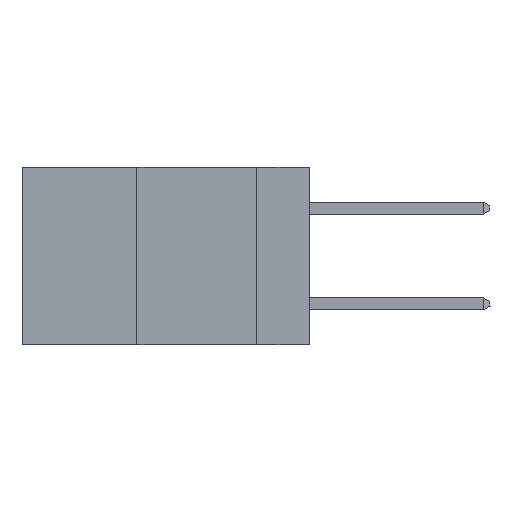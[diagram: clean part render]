
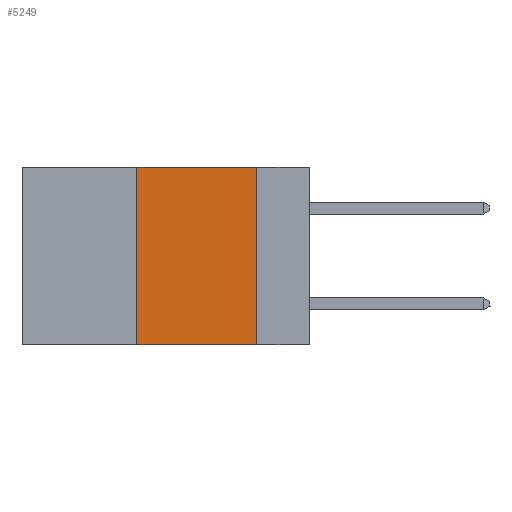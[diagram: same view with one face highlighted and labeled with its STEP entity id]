
A CAD part, left-side view. The second image highlights one B-rep face of the part: STEP entity #5249.
In plain terms, the highlighted planar face has unit normal (-1, 0, 0).
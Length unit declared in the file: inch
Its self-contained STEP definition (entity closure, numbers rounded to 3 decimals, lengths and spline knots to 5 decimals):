
#216 = AXIS2_PLACEMENT_3D ( 'NONE', #523, #10681, #2516 ) ;
#227 = CARTESIAN_POINT ( 'NONE',  ( 0., 0.36, 0. ) ) ;
#523 = CARTESIAN_POINT ( 'NONE',  ( 0., 0.6, 0. ) ) ;
#568 = VECTOR ( 'NONE', #9889, 39.37008 ) ;
#1484 = CARTESIAN_POINT ( 'NONE',  ( 0., 0.36, -0.37 ) ) ;
#1761 = DIRECTION ( 'NONE',  ( 0., 0., 1. ) ) ;
#1946 = LINE ( 'NONE', #11132, #568 ) ;
#2516 = DIRECTION ( 'NONE',  ( 0., 0., -1. ) ) ;
#2603 = EDGE_CURVE ( 'NONE', #17367, #16908, #8984, .T. ) ;
#2927 = VECTOR ( 'NONE', #9873, 39.37008 ) ;
#3128 = VECTOR ( 'NONE', #1761, 39.37008 ) ;
#3724 = ORIENTED_EDGE ( 'NONE', *, *, #2603, .F. ) ;
#4278 = ORIENTED_EDGE ( 'NONE', *, *, #18104, .F. ) ;
#4289 = VECTOR ( 'NONE', #13635, 39.37008 ) ;
#4836 = CARTESIAN_POINT ( 'NONE',  ( 0., 0.36, 0. ) ) ;
#5249 = ADVANCED_FACE ( 'NONE', ( #7454 ), #11201, .F. ) ;
#5615 = LINE ( 'NONE', #10708, #4289 ) ;
#5779 = EDGE_CURVE ( 'NONE', #17367, #15905, #10385, .T. ) ;
#6176 = CARTESIAN_POINT ( 'NONE',  ( 0., 0.11, -0.37 ) ) ;
#7238 = EDGE_CURVE ( 'NONE', #7621, #15905, #1946, .T. ) ;
#7251 = CARTESIAN_POINT ( 'NONE',  ( 0., 0.11, 0. ) ) ;
#7454 = FACE_OUTER_BOUND ( 'NONE', #12833, .T. ) ;
#7621 = VERTEX_POINT ( 'NONE', #7251 ) ;
#8984 = LINE ( 'NONE', #227, #3128 ) ;
#9220 = ORIENTED_EDGE ( 'NONE', *, *, #5779, .T. ) ;
#9873 = DIRECTION ( 'NONE',  ( 0., -1., 0. ) ) ;
#9889 = DIRECTION ( 'NONE',  ( 0., 0., -1. ) ) ;
#10385 = LINE ( 'NONE', #18572, #2927 ) ;
#10681 = DIRECTION ( 'NONE',  ( 1., 0., 0. ) ) ;
#10708 = CARTESIAN_POINT ( 'NONE',  ( 0., 0.6, 0. ) ) ;
#11132 = CARTESIAN_POINT ( 'NONE',  ( 0., 0.11, 0. ) ) ;
#11201 = PLANE ( 'NONE',  #216 ) ;
#12833 = EDGE_LOOP ( 'NONE', ( #15552, #4278, #3724, #9220 ) ) ;
#13635 = DIRECTION ( 'NONE',  ( 0., -1., 0. ) ) ;
#15552 = ORIENTED_EDGE ( 'NONE', *, *, #7238, .F. ) ;
#15905 = VERTEX_POINT ( 'NONE', #6176 ) ;
#16908 = VERTEX_POINT ( 'NONE', #4836 ) ;
#17367 = VERTEX_POINT ( 'NONE', #1484 ) ;
#18104 = EDGE_CURVE ( 'NONE', #16908, #7621, #5615, .T. ) ;
#18572 = CARTESIAN_POINT ( 'NONE',  ( 0., 0.6, -0.37 ) ) ;
